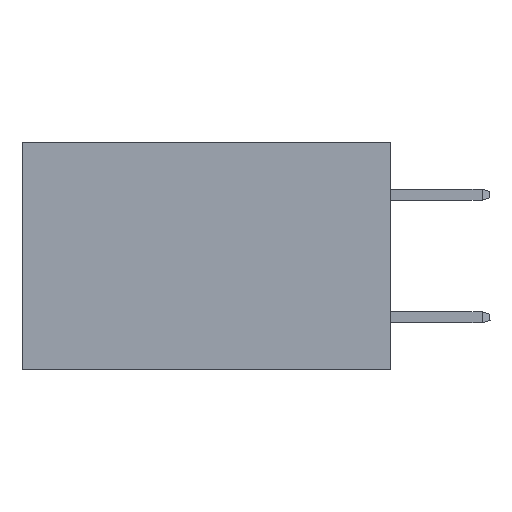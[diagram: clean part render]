
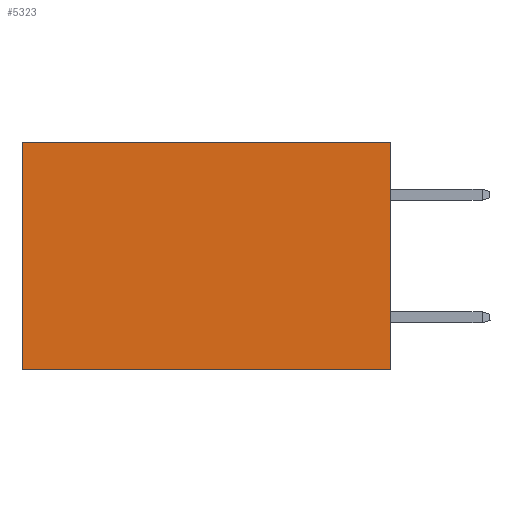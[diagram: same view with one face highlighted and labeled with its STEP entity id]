
A CAD part, left-side view. The second image highlights one B-rep face of the part: STEP entity #5323.
In plain terms, the highlighted planar face has unit normal (-1, 0, 0).
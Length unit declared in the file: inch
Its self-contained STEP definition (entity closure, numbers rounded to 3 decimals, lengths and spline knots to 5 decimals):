
#276 = LINE ( 'NONE', #4191, #19440 ) ;
#316 = CARTESIAN_POINT ( 'NONE',  ( 0.2875, 0., -0.37 ) ) ;
#416 = EDGE_CURVE ( 'NONE', #14989, #6106, #276, .T. ) ;
#652 = EDGE_CURVE ( 'NONE', #7525, #13908, #3948, .T. ) ;
#979 = VECTOR ( 'NONE', #11642, 39.37008 ) ;
#1099 = CARTESIAN_POINT ( 'NONE',  ( 0.2875, 0.6, 0. ) ) ;
#2144 = ORIENTED_EDGE ( 'NONE', *, *, #652, .F. ) ;
#2356 = VECTOR ( 'NONE', #6789, 39.37008 ) ;
#2475 = CARTESIAN_POINT ( 'NONE',  ( 0.2875, 0., 0. ) ) ;
#2561 = ORIENTED_EDGE ( 'NONE', *, *, #10999, .T. ) ;
#3948 = LINE ( 'NONE', #18385, #2356 ) ;
#4130 = CARTESIAN_POINT ( 'NONE',  ( 0.2875, 0., 0. ) ) ;
#4191 = CARTESIAN_POINT ( 'NONE',  ( 0.2875, 0.6, 0. ) ) ;
#4424 = EDGE_CURVE ( 'NONE', #13908, #6106, #11100, .T. ) ;
#5323 = ADVANCED_FACE ( 'NONE', ( #14642 ), #11799, .F. ) ;
#6106 = VERTEX_POINT ( 'NONE', #19725 ) ;
#6648 = DIRECTION ( 'NONE',  ( 0., 0., -1. ) ) ;
#6789 = DIRECTION ( 'NONE',  ( 0., 0., -1. ) ) ;
#7525 = VERTEX_POINT ( 'NONE', #4130 ) ;
#8193 = AXIS2_PLACEMENT_3D ( 'NONE', #11027, #19844, #6648 ) ;
#8603 = LINE ( 'NONE', #2475, #979 ) ;
#9301 = DIRECTION ( 'NONE',  ( 0., 0., -1. ) ) ;
#10309 = ORIENTED_EDGE ( 'NONE', *, *, #4424, .F. ) ;
#10999 = EDGE_CURVE ( 'NONE', #7525, #14989, #8603, .T. ) ;
#11027 = CARTESIAN_POINT ( 'NONE',  ( 0.2875, 0., 0. ) ) ;
#11100 = LINE ( 'NONE', #316, #11367 ) ;
#11367 = VECTOR ( 'NONE', #15458, 39.37008 ) ;
#11642 = DIRECTION ( 'NONE',  ( 0., 1., 0. ) ) ;
#11799 = PLANE ( 'NONE',  #8193 ) ;
#13908 = VERTEX_POINT ( 'NONE', #14115 ) ;
#14115 = CARTESIAN_POINT ( 'NONE',  ( 0.2875, 0., -0.37 ) ) ;
#14158 = ORIENTED_EDGE ( 'NONE', *, *, #416, .T. ) ;
#14642 = FACE_OUTER_BOUND ( 'NONE', #16441, .T. ) ;
#14989 = VERTEX_POINT ( 'NONE', #1099 ) ;
#15458 = DIRECTION ( 'NONE',  ( 0., 1., 0. ) ) ;
#16441 = EDGE_LOOP ( 'NONE', ( #14158, #10309, #2144, #2561 ) ) ;
#18385 = CARTESIAN_POINT ( 'NONE',  ( 0.2875, 0., 0. ) ) ;
#19440 = VECTOR ( 'NONE', #9301, 39.37008 ) ;
#19725 = CARTESIAN_POINT ( 'NONE',  ( 0.2875, 0.6, -0.37 ) ) ;
#19844 = DIRECTION ( 'NONE',  ( 1., 0., 0. ) ) ;
